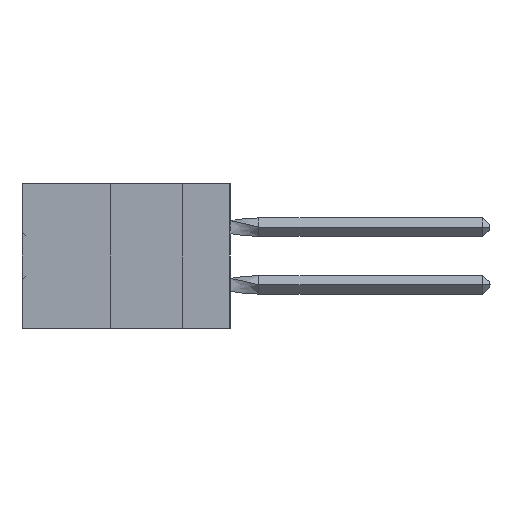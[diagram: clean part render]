
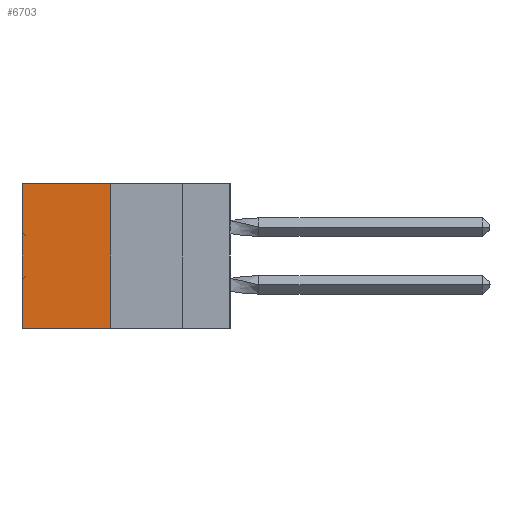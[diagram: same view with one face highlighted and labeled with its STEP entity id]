
A CAD part, left-side view. The second image highlights one B-rep face of the part: STEP entity #6703.
In plain terms, the highlighted planar face has unit normal (-1, 0, 0).
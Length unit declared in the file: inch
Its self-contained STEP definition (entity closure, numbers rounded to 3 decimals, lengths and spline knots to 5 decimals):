
#3030 = VERTEX_POINT ( 'NONE', #47117 ) ;
#3458 = CARTESIAN_POINT ( 'NONE',  ( 0.305, 0.413, 0. ) ) ;
#4063 = ORIENTED_EDGE ( 'NONE', *, *, #28932, .T. ) ;
#5047 = CARTESIAN_POINT ( 'NONE',  ( 0.305, 0.413, 0. ) ) ;
#6681 = CARTESIAN_POINT ( 'NONE',  ( 0.305, 0.413, -0.5 ) ) ;
#6703 = ADVANCED_FACE ( 'NONE', ( #63101 ), #24897, .F. ) ;
#8970 = VECTOR ( 'NONE', #54853, 39.37008 ) ;
#10821 = EDGE_CURVE ( 'NONE', #45540, #20789, #49418, .T. ) ;
#11849 = LINE ( 'NONE', #3458, #15643 ) ;
#12526 = AXIS2_PLACEMENT_3D ( 'NONE', #43637, #19347, #19120 ) ;
#15643 = VECTOR ( 'NONE', #18382, 39.37008 ) ;
#18382 = DIRECTION ( 'NONE',  ( 0., 1., 0. ) ) ;
#18457 = VECTOR ( 'NONE', #49144, 39.37008 ) ;
#19120 = DIRECTION ( 'NONE',  ( 0., 0., -1. ) ) ;
#19347 = DIRECTION ( 'NONE',  ( 1., 0., 0. ) ) ;
#19837 = DIRECTION ( 'NONE',  ( 0., 1., 0. ) ) ;
#20771 = CARTESIAN_POINT ( 'NONE',  ( 0.305, 0.413, -0.5 ) ) ;
#20789 = VERTEX_POINT ( 'NONE', #6681 ) ;
#21699 = ORIENTED_EDGE ( 'NONE', *, *, #49131, .T. ) ;
#24897 = PLANE ( 'NONE',  #12526 ) ;
#28932 = EDGE_CURVE ( 'NONE', #53833, #3030, #31469, .T. ) ;
#28998 = CARTESIAN_POINT ( 'NONE',  ( 0.305, 0.72, 0. ) ) ;
#29983 = CARTESIAN_POINT ( 'NONE',  ( 0.305, 0.72, -0.5 ) ) ;
#30487 = LINE ( 'NONE', #38363, #54857 ) ;
#31469 = LINE ( 'NONE', #29983, #18457 ) ;
#36966 = ORIENTED_EDGE ( 'NONE', *, *, #42809, .F. ) ;
#38363 = CARTESIAN_POINT ( 'NONE',  ( 0.305, 0.413, -0.5 ) ) ;
#42809 = EDGE_CURVE ( 'NONE', #20789, #3030, #30487, .T. ) ;
#43617 = ORIENTED_EDGE ( 'NONE', *, *, #10821, .F. ) ;
#43637 = CARTESIAN_POINT ( 'NONE',  ( 0.305, 0.413, -0.5 ) ) ;
#45540 = VERTEX_POINT ( 'NONE', #5047 ) ;
#45926 = EDGE_LOOP ( 'NONE', ( #4063, #36966, #43617, #21699 ) ) ;
#47117 = CARTESIAN_POINT ( 'NONE',  ( 0.305, 0.72, -0.5 ) ) ;
#49131 = EDGE_CURVE ( 'NONE', #45540, #53833, #11849, .T. ) ;
#49144 = DIRECTION ( 'NONE',  ( 0., 0., -1. ) ) ;
#49418 = LINE ( 'NONE', #20771, #8970 ) ;
#53833 = VERTEX_POINT ( 'NONE', #28998 ) ;
#54853 = DIRECTION ( 'NONE',  ( 0., 0., -1. ) ) ;
#54857 = VECTOR ( 'NONE', #19837, 39.37008 ) ;
#63101 = FACE_OUTER_BOUND ( 'NONE', #45926, .T. ) ;
